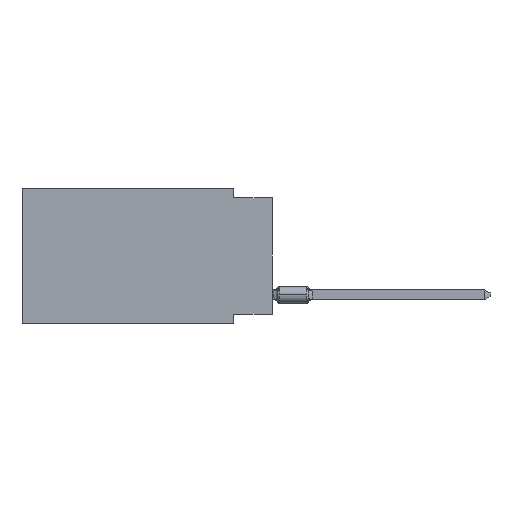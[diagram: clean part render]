
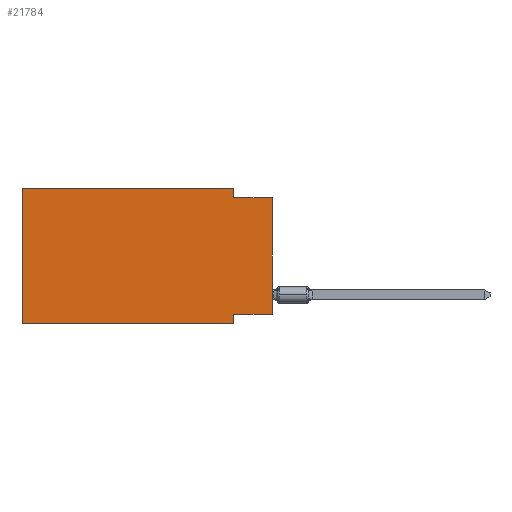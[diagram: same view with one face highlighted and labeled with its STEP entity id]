
A CAD part, left-side view. The second image highlights one B-rep face of the part: STEP entity #21784.
In plain terms, the highlighted planar face has unit normal (-1, 0, 0).
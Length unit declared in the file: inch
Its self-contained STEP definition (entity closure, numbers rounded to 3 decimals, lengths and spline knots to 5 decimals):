
#1306 = DIRECTION ( 'NONE',  ( 0., 0., -1. ) ) ;
#1579 = DIRECTION ( 'NONE',  ( 0., 0., 1. ) ) ;
#2227 = CARTESIAN_POINT ( 'NONE',  ( 0., 0., -0.025 ) ) ;
#2712 = CARTESIAN_POINT ( 'NONE',  ( 0., 0.1, -0.325 ) ) ;
#2818 = VECTOR ( 'NONE', #1579, 39.37008 ) ;
#2895 = CARTESIAN_POINT ( 'NONE',  ( 0., 0.1, -0.35 ) ) ;
#3190 = LINE ( 'NONE', #4253, #6863 ) ;
#3629 = LINE ( 'NONE', #3857, #9440 ) ;
#3857 = CARTESIAN_POINT ( 'NONE',  ( 0., 0.645, -0.35 ) ) ;
#3893 = CARTESIAN_POINT ( 'NONE',  ( 0., 0.645, 0. ) ) ;
#4253 = CARTESIAN_POINT ( 'NONE',  ( 0., 0.1, -0.35 ) ) ;
#4783 = ORIENTED_EDGE ( 'NONE', *, *, #17410, .F. ) ;
#4789 = CARTESIAN_POINT ( 'NONE',  ( 0., 0.645, 0. ) ) ;
#5129 = CARTESIAN_POINT ( 'NONE',  ( 0., 0.1, 0. ) ) ;
#5282 = ORIENTED_EDGE ( 'NONE', *, *, #10072, .T. ) ;
#5601 = ORIENTED_EDGE ( 'NONE', *, *, #13680, .F. ) ;
#6339 = VERTEX_POINT ( 'NONE', #18384 ) ;
#6481 = CARTESIAN_POINT ( 'NONE',  ( 0., 0.1, 0. ) ) ;
#6531 = EDGE_CURVE ( 'NONE', #18184, #20376, #17330, .T. ) ;
#6538 = VECTOR ( 'NONE', #12715, 39.37008 ) ;
#6631 = DIRECTION ( 'NONE',  ( 1., 0., 0. ) ) ;
#6863 = VECTOR ( 'NONE', #17010, 39.37008 ) ;
#6940 = LINE ( 'NONE', #2227, #15032 ) ;
#7009 = EDGE_CURVE ( 'NONE', #6339, #15518, #6940, .T. ) ;
#7140 = DIRECTION ( 'NONE',  ( 0., 1., 0. ) ) ;
#7391 = DIRECTION ( 'NONE',  ( 0., -1., 0. ) ) ;
#7886 = LINE ( 'NONE', #3893, #13535 ) ;
#8077 = CARTESIAN_POINT ( 'NONE',  ( 0., 0., -0.025 ) ) ;
#8592 = VERTEX_POINT ( 'NONE', #5129 ) ;
#9440 = VECTOR ( 'NONE', #17682, 39.37008 ) ;
#10072 = EDGE_CURVE ( 'NONE', #17747, #15518, #17099, .T. ) ;
#10308 = CARTESIAN_POINT ( 'NONE',  ( 0., 0., 0. ) ) ;
#10387 = EDGE_LOOP ( 'NONE', ( #5282, #21467, #11676, #4783, #17480, #21578, #5601, #21740 ) ) ;
#10814 = LINE ( 'NONE', #15999, #17871 ) ;
#10851 = CARTESIAN_POINT ( 'NONE',  ( 0., 0., -0.325 ) ) ;
#11469 = DIRECTION ( 'NONE',  ( 0., -1., 0. ) ) ;
#11676 = ORIENTED_EDGE ( 'NONE', *, *, #22046, .F. ) ;
#11816 = DIRECTION ( 'NONE',  ( 0., 0., -1. ) ) ;
#12715 = DIRECTION ( 'NONE',  ( 0., 0., 1. ) ) ;
#12825 = AXIS2_PLACEMENT_3D ( 'NONE', #4789, #6631, #11816 ) ;
#12924 = CARTESIAN_POINT ( 'NONE',  ( 0., 0.645, -0.35 ) ) ;
#13535 = VECTOR ( 'NONE', #11469, 39.37008 ) ;
#13542 = EDGE_CURVE ( 'NONE', #17747, #22158, #10814, .T. ) ;
#13680 = EDGE_CURVE ( 'NONE', #22158, #17150, #3190, .T. ) ;
#15032 = VECTOR ( 'NONE', #7391, 39.37008 ) ;
#15502 = PLANE ( 'NONE',  #12825 ) ;
#15518 = VERTEX_POINT ( 'NONE', #8077 ) ;
#15850 = CARTESIAN_POINT ( 'NONE',  ( 0., 0.645, 0. ) ) ;
#15999 = CARTESIAN_POINT ( 'NONE',  ( 0., 0., -0.325 ) ) ;
#16126 = EDGE_CURVE ( 'NONE', #18184, #17150, #3629, .T. ) ;
#17010 = DIRECTION ( 'NONE',  ( 0., 0., -1. ) ) ;
#17071 = LINE ( 'NONE', #6481, #18288 ) ;
#17099 = LINE ( 'NONE', #10308, #2818 ) ;
#17150 = VERTEX_POINT ( 'NONE', #2895 ) ;
#17330 = LINE ( 'NONE', #21222, #6538 ) ;
#17410 = EDGE_CURVE ( 'NONE', #20376, #8592, #7886, .T. ) ;
#17480 = ORIENTED_EDGE ( 'NONE', *, *, #6531, .F. ) ;
#17682 = DIRECTION ( 'NONE',  ( 0., -1., 0. ) ) ;
#17747 = VERTEX_POINT ( 'NONE', #10851 ) ;
#17871 = VECTOR ( 'NONE', #7140, 39.37008 ) ;
#18184 = VERTEX_POINT ( 'NONE', #12924 ) ;
#18288 = VECTOR ( 'NONE', #1306, 39.37008 ) ;
#18384 = CARTESIAN_POINT ( 'NONE',  ( 0., 0.1, -0.025 ) ) ;
#20376 = VERTEX_POINT ( 'NONE', #15850 ) ;
#20559 = FACE_OUTER_BOUND ( 'NONE', #10387, .T. ) ;
#21222 = CARTESIAN_POINT ( 'NONE',  ( 0., 0.645, 0. ) ) ;
#21467 = ORIENTED_EDGE ( 'NONE', *, *, #7009, .F. ) ;
#21578 = ORIENTED_EDGE ( 'NONE', *, *, #16126, .T. ) ;
#21740 = ORIENTED_EDGE ( 'NONE', *, *, #13542, .F. ) ;
#21784 = ADVANCED_FACE ( 'NONE', ( #20559 ), #15502, .F. ) ;
#22046 = EDGE_CURVE ( 'NONE', #8592, #6339, #17071, .T. ) ;
#22158 = VERTEX_POINT ( 'NONE', #2712 ) ;
